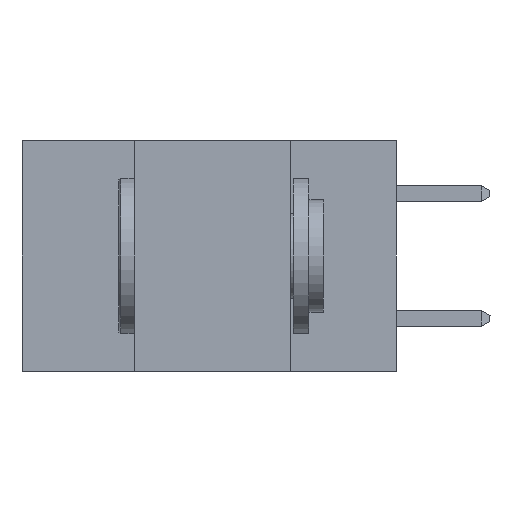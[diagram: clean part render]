
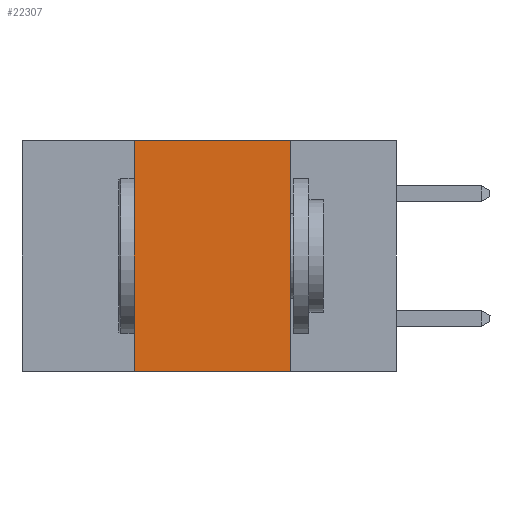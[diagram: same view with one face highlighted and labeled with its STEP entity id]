
A CAD part, left-side view. The second image highlights one B-rep face of the part: STEP entity #22307.
In plain terms, the highlighted planar face has unit normal (-1, 0, 0).
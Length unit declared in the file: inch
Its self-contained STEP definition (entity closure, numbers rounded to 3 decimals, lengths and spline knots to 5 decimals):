
#61 = VECTOR ( 'NONE', #7636, 39.37008 ) ;
#81 = ORIENTED_EDGE ( 'NONE', *, *, #14265, .T. ) ;
#1181 = VERTEX_POINT ( 'NONE', #7595 ) ;
#2396 = PLANE ( 'NONE',  #3056 ) ;
#2485 = LINE ( 'NONE', #5819, #7124 ) ;
#3056 = AXIS2_PLACEMENT_3D ( 'NONE', #12328, #16245, #4367 ) ;
#3355 = LINE ( 'NONE', #12554, #18482 ) ;
#3407 = VECTOR ( 'NONE', #21730, 39.37008 ) ;
#3660 = CARTESIAN_POINT ( 'NONE',  ( 0., 0.6, -0.37 ) ) ;
#3949 = EDGE_LOOP ( 'NONE', ( #6348, #5715, #22447, #81 ) ) ;
#4367 = DIRECTION ( 'NONE',  ( 0., 0., -1. ) ) ;
#5298 = VERTEX_POINT ( 'NONE', #17348 ) ;
#5715 = ORIENTED_EDGE ( 'NONE', *, *, #17379, .F. ) ;
#5819 = CARTESIAN_POINT ( 'NONE',  ( 0., 0.42, -0.37 ) ) ;
#6348 = ORIENTED_EDGE ( 'NONE', *, *, #18271, .F. ) ;
#7124 = VECTOR ( 'NONE', #21503, 39.37008 ) ;
#7595 = CARTESIAN_POINT ( 'NONE',  ( 0., 0.17, -0.37 ) ) ;
#7636 = DIRECTION ( 'NONE',  ( 0., -1., 0. ) ) ;
#12328 = CARTESIAN_POINT ( 'NONE',  ( 0., 0.6, 0. ) ) ;
#12554 = CARTESIAN_POINT ( 'NONE',  ( 0., 0.17, -0.37 ) ) ;
#12603 = CARTESIAN_POINT ( 'NONE',  ( 0., 0.42, 0. ) ) ;
#13445 = EDGE_CURVE ( 'NONE', #5298, #23684, #2485, .T. ) ;
#14028 = CARTESIAN_POINT ( 'NONE',  ( 0., 0.6, 0. ) ) ;
#14265 = EDGE_CURVE ( 'NONE', #5298, #1181, #15825, .T. ) ;
#14688 = FACE_OUTER_BOUND ( 'NONE', #3949, .T. ) ;
#15825 = LINE ( 'NONE', #3660, #61 ) ;
#16245 = DIRECTION ( 'NONE',  ( 1., 0., 0. ) ) ;
#16345 = VERTEX_POINT ( 'NONE', #23535 ) ;
#17348 = CARTESIAN_POINT ( 'NONE',  ( 0., 0.42, -0.37 ) ) ;
#17379 = EDGE_CURVE ( 'NONE', #23684, #16345, #23045, .T. ) ;
#18271 = EDGE_CURVE ( 'NONE', #16345, #1181, #3355, .T. ) ;
#18482 = VECTOR ( 'NONE', #24093, 39.37008 ) ;
#21503 = DIRECTION ( 'NONE',  ( 0., 0., 1. ) ) ;
#21730 = DIRECTION ( 'NONE',  ( 0., -1., 0. ) ) ;
#22307 = ADVANCED_FACE ( 'NONE', ( #14688 ), #2396, .F. ) ;
#22447 = ORIENTED_EDGE ( 'NONE', *, *, #13445, .F. ) ;
#23045 = LINE ( 'NONE', #14028, #3407 ) ;
#23535 = CARTESIAN_POINT ( 'NONE',  ( 0., 0.17, 0. ) ) ;
#23684 = VERTEX_POINT ( 'NONE', #12603 ) ;
#24093 = DIRECTION ( 'NONE',  ( 0., 0., -1. ) ) ;
